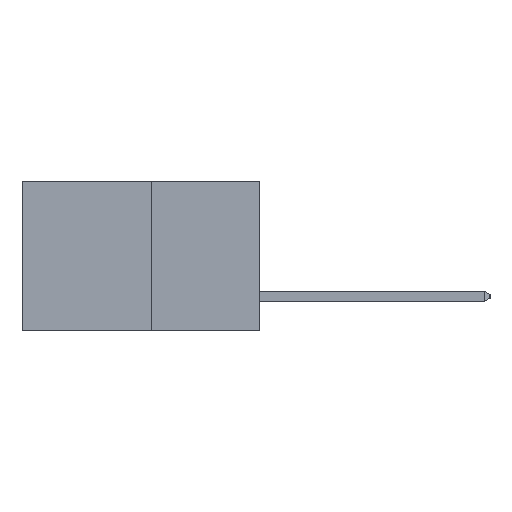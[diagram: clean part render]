
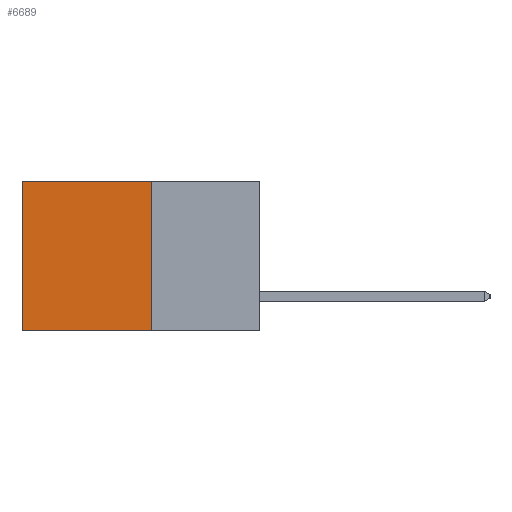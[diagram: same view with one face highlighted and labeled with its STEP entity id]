
A CAD part, left-side view. The second image highlights one B-rep face of the part: STEP entity #6689.
In plain terms, the highlighted planar face has unit normal (-1, 0, 0).
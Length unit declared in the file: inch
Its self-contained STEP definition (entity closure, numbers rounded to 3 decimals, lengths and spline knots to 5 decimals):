
#246 = FACE_OUTER_BOUND ( 'NONE', #8786, .T. ) ;
#385 = VERTEX_POINT ( 'NONE', #7907 ) ;
#514 = DIRECTION ( 'NONE',  ( 0., 1., 0. ) ) ;
#526 = LINE ( 'NONE', #7414, #8979 ) ;
#527 = CARTESIAN_POINT ( 'NONE',  ( 0.277, 0.27, -0.37 ) ) ;
#649 = VERTEX_POINT ( 'NONE', #10222 ) ;
#4173 = ORIENTED_EDGE ( 'NONE', *, *, #12762, .T. ) ;
#4476 = EDGE_CURVE ( 'NONE', #649, #10114, #526, .T. ) ;
#5637 = VERTEX_POINT ( 'NONE', #11992 ) ;
#6689 = ADVANCED_FACE ( 'NONE', ( #246 ), #13043, .F. ) ;
#7022 = AXIS2_PLACEMENT_3D ( 'NONE', #10175, #12754, #12735 ) ;
#7414 = CARTESIAN_POINT ( 'NONE',  ( 0.277, 0.59, -0.37 ) ) ;
#7907 = CARTESIAN_POINT ( 'NONE',  ( 0.277, 0.27, 0. ) ) ;
#7927 = EDGE_CURVE ( 'NONE', #5637, #10114, #11896, .T. ) ;
#7963 = ORIENTED_EDGE ( 'NONE', *, *, #4476, .T. ) ;
#8216 = CARTESIAN_POINT ( 'NONE',  ( 0.277, 0.27, -0.37 ) ) ;
#8294 = ORIENTED_EDGE ( 'NONE', *, *, #10878, .F. ) ;
#8786 = EDGE_LOOP ( 'NONE', ( #7963, #12605, #8294, #4173 ) ) ;
#8810 = CARTESIAN_POINT ( 'NONE',  ( 0.277, 0.59, -0.37 ) ) ;
#8979 = VECTOR ( 'NONE', #10520, 39.37008 ) ;
#9518 = VECTOR ( 'NONE', #10903, 39.37008 ) ;
#9820 = LINE ( 'NONE', #9896, #9518 ) ;
#9896 = CARTESIAN_POINT ( 'NONE',  ( 0.277, 0.27, 0. ) ) ;
#10114 = VERTEX_POINT ( 'NONE', #8810 ) ;
#10175 = CARTESIAN_POINT ( 'NONE',  ( 0.277, 0.27, -0.37 ) ) ;
#10184 = VECTOR ( 'NONE', #10227, 39.37008 ) ;
#10222 = CARTESIAN_POINT ( 'NONE',  ( 0.277, 0.59, 0. ) ) ;
#10227 = DIRECTION ( 'NONE',  ( 0., 0., -1. ) ) ;
#10520 = DIRECTION ( 'NONE',  ( 0., 0., -1. ) ) ;
#10878 = EDGE_CURVE ( 'NONE', #385, #5637, #12760, .T. ) ;
#10903 = DIRECTION ( 'NONE',  ( 0., 1., 0. ) ) ;
#11896 = LINE ( 'NONE', #527, #12204 ) ;
#11992 = CARTESIAN_POINT ( 'NONE',  ( 0.277, 0.27, -0.37 ) ) ;
#12204 = VECTOR ( 'NONE', #514, 39.37008 ) ;
#12605 = ORIENTED_EDGE ( 'NONE', *, *, #7927, .F. ) ;
#12735 = DIRECTION ( 'NONE',  ( 0., 0., -1. ) ) ;
#12754 = DIRECTION ( 'NONE',  ( 1., 0., 0. ) ) ;
#12760 = LINE ( 'NONE', #8216, #10184 ) ;
#12762 = EDGE_CURVE ( 'NONE', #385, #649, #9820, .T. ) ;
#13043 = PLANE ( 'NONE',  #7022 ) ;
